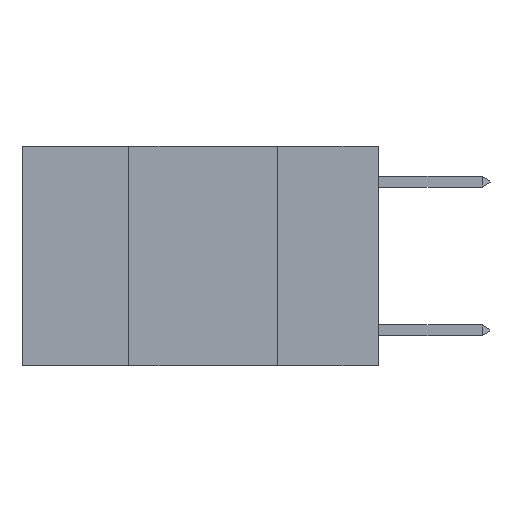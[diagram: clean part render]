
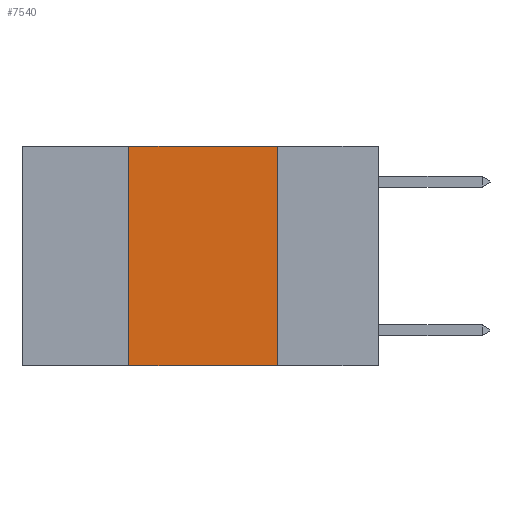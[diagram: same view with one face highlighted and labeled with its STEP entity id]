
A CAD part, left-side view. The second image highlights one B-rep face of the part: STEP entity #7540.
In plain terms, the highlighted planar face has unit normal (-1, 0, 0).
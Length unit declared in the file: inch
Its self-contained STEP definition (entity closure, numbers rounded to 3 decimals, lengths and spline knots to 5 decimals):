
#47 = VECTOR ( 'NONE', #7547, 39.37008 ) ;
#266 = LINE ( 'NONE', #5226, #3483 ) ;
#343 = CARTESIAN_POINT ( 'NONE',  ( 0., 0.17, 0. ) ) ;
#563 = DIRECTION ( 'NONE',  ( 0., 0., 1. ) ) ;
#752 = LINE ( 'NONE', #7511, #14158 ) ;
#1510 = ORIENTED_EDGE ( 'NONE', *, *, #2945, .F. ) ;
#1896 = CARTESIAN_POINT ( 'NONE',  ( 0., 0.42, 0. ) ) ;
#2242 = DIRECTION ( 'NONE',  ( 0., -1., 0. ) ) ;
#2660 = EDGE_LOOP ( 'NONE', ( #13851, #1510, #3589, #8178 ) ) ;
#2945 = EDGE_CURVE ( 'NONE', #7285, #8639, #752, .T. ) ;
#3470 = DIRECTION ( 'NONE',  ( 1., 0., 0. ) ) ;
#3483 = VECTOR ( 'NONE', #6600, 39.37008 ) ;
#3589 = ORIENTED_EDGE ( 'NONE', *, *, #6958, .F. ) ;
#3776 = EDGE_CURVE ( 'NONE', #5437, #6133, #4091, .T. ) ;
#3995 = EDGE_CURVE ( 'NONE', #8639, #6133, #266, .T. ) ;
#4091 = LINE ( 'NONE', #11311, #47 ) ;
#4334 = FACE_OUTER_BOUND ( 'NONE', #2660, .T. ) ;
#5226 = CARTESIAN_POINT ( 'NONE',  ( 0., 0.17, 0. ) ) ;
#5437 = VERTEX_POINT ( 'NONE', #10817 ) ;
#5566 = CARTESIAN_POINT ( 'NONE',  ( 0., 0.42, 0. ) ) ;
#6133 = VERTEX_POINT ( 'NONE', #16630 ) ;
#6600 = DIRECTION ( 'NONE',  ( 0., 0., -1. ) ) ;
#6958 = EDGE_CURVE ( 'NONE', #5437, #7285, #13616, .T. ) ;
#7285 = VERTEX_POINT ( 'NONE', #5566 ) ;
#7401 = CARTESIAN_POINT ( 'NONE',  ( 0., 0.6, 0. ) ) ;
#7511 = CARTESIAN_POINT ( 'NONE',  ( 0., 0.6, 0. ) ) ;
#7540 = ADVANCED_FACE ( 'NONE', ( #4334 ), #10002, .F. ) ;
#7547 = DIRECTION ( 'NONE',  ( 0., -1., 0. ) ) ;
#8178 = ORIENTED_EDGE ( 'NONE', *, *, #3776, .T. ) ;
#8639 = VERTEX_POINT ( 'NONE', #343 ) ;
#9338 = AXIS2_PLACEMENT_3D ( 'NONE', #7401, #3470, #12507 ) ;
#10002 = PLANE ( 'NONE',  #9338 ) ;
#10297 = VECTOR ( 'NONE', #563, 39.37008 ) ;
#10817 = CARTESIAN_POINT ( 'NONE',  ( 0., 0.42, -0.37 ) ) ;
#11311 = CARTESIAN_POINT ( 'NONE',  ( 0., 0.6, -0.37 ) ) ;
#12507 = DIRECTION ( 'NONE',  ( 0., 0., -1. ) ) ;
#13616 = LINE ( 'NONE', #1896, #10297 ) ;
#13851 = ORIENTED_EDGE ( 'NONE', *, *, #3995, .F. ) ;
#14158 = VECTOR ( 'NONE', #2242, 39.37008 ) ;
#16630 = CARTESIAN_POINT ( 'NONE',  ( 0., 0.17, -0.37 ) ) ;
